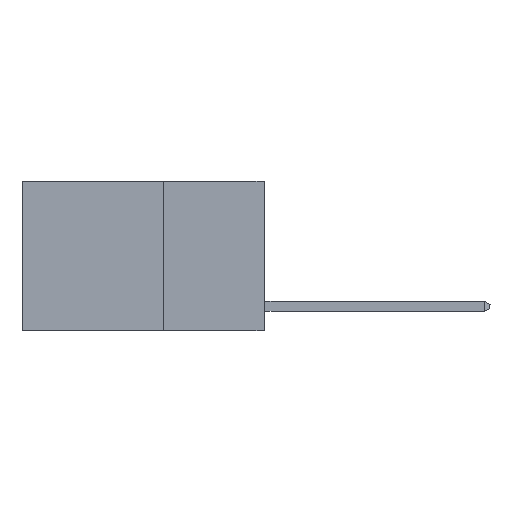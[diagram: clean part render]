
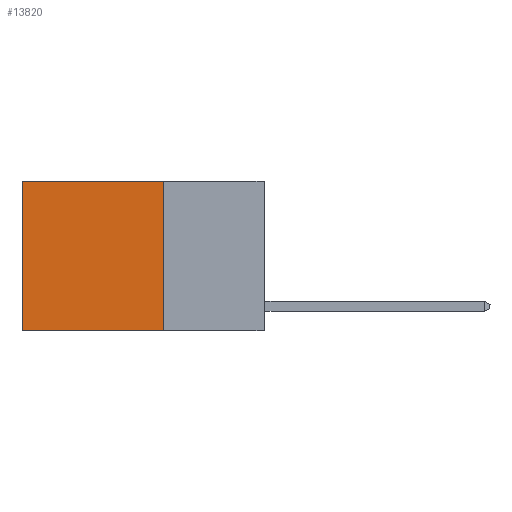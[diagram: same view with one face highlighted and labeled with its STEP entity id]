
A CAD part, left-side view. The second image highlights one B-rep face of the part: STEP entity #13820.
In plain terms, the highlighted planar face has unit normal (-1, 0, 0).
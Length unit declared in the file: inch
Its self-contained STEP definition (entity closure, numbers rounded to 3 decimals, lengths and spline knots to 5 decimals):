
#469 = EDGE_CURVE ( 'NONE', #7750, #7333, #4575, .T. ) ;
#573 = CARTESIAN_POINT ( 'NONE',  ( 0.2625, 0.25, 0. ) ) ;
#695 = EDGE_CURVE ( 'NONE', #10226, #13878, #2511, .T. ) ;
#1528 = LINE ( 'NONE', #9926, #7099 ) ;
#1564 = CARTESIAN_POINT ( 'NONE',  ( 0.2625, 0.6, 0. ) ) ;
#1594 = VECTOR ( 'NONE', #2466, 39.37008 ) ;
#2093 = EDGE_CURVE ( 'NONE', #13878, #7333, #13300, .T. ) ;
#2154 = VECTOR ( 'NONE', #4907, 39.37008 ) ;
#2378 = EDGE_CURVE ( 'NONE', #10226, #7750, #1528, .T. ) ;
#2417 = CARTESIAN_POINT ( 'NONE',  ( 0.2625, 0.6, 0. ) ) ;
#2466 = DIRECTION ( 'NONE',  ( 0., 0., -1. ) ) ;
#2511 = LINE ( 'NONE', #10408, #2154 ) ;
#3171 = ORIENTED_EDGE ( 'NONE', *, *, #695, .F. ) ;
#4063 = CARTESIAN_POINT ( 'NONE',  ( 0.2625, 0.25, -0.37 ) ) ;
#4575 = LINE ( 'NONE', #2417, #1594 ) ;
#4709 = VECTOR ( 'NONE', #5174, 39.37008 ) ;
#4858 = ORIENTED_EDGE ( 'NONE', *, *, #469, .T. ) ;
#4907 = DIRECTION ( 'NONE',  ( 0., 0., -1. ) ) ;
#5113 = PLANE ( 'NONE',  #12619 ) ;
#5174 = DIRECTION ( 'NONE',  ( 0., 1., 0. ) ) ;
#5614 = DIRECTION ( 'NONE',  ( 0., 1., 0. ) ) ;
#6141 = CARTESIAN_POINT ( 'NONE',  ( 0.2625, 0.25, 0. ) ) ;
#6235 = DIRECTION ( 'NONE',  ( 1., 0., 0. ) ) ;
#7099 = VECTOR ( 'NONE', #5614, 39.37008 ) ;
#7121 = ORIENTED_EDGE ( 'NONE', *, *, #2093, .F. ) ;
#7333 = VERTEX_POINT ( 'NONE', #12881 ) ;
#7389 = EDGE_LOOP ( 'NONE', ( #4858, #7121, #3171, #8615 ) ) ;
#7673 = FACE_OUTER_BOUND ( 'NONE', #7389, .T. ) ;
#7750 = VERTEX_POINT ( 'NONE', #1564 ) ;
#8615 = ORIENTED_EDGE ( 'NONE', *, *, #2378, .T. ) ;
#9926 = CARTESIAN_POINT ( 'NONE',  ( 0.2625, 0.25, 0. ) ) ;
#10226 = VERTEX_POINT ( 'NONE', #6141 ) ;
#10408 = CARTESIAN_POINT ( 'NONE',  ( 0.2625, 0.25, 0. ) ) ;
#11732 = CARTESIAN_POINT ( 'NONE',  ( 0.2625, 0.25, -0.37 ) ) ;
#12619 = AXIS2_PLACEMENT_3D ( 'NONE', #573, #6235, #13701 ) ;
#12881 = CARTESIAN_POINT ( 'NONE',  ( 0.2625, 0.6, -0.37 ) ) ;
#13300 = LINE ( 'NONE', #4063, #4709 ) ;
#13701 = DIRECTION ( 'NONE',  ( 0., 0., -1. ) ) ;
#13820 = ADVANCED_FACE ( 'NONE', ( #7673 ), #5113, .F. ) ;
#13878 = VERTEX_POINT ( 'NONE', #11732 ) ;
